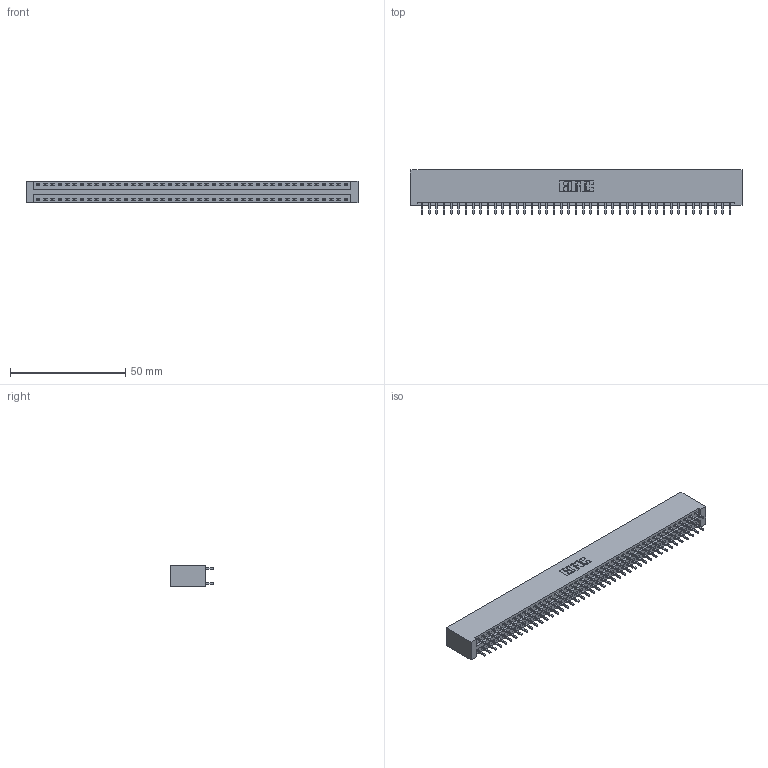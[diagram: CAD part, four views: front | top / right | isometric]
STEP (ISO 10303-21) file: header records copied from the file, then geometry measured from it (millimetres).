
FILE_DESCRIPTION (( 'STEP AP203' ), '1' );
FILE_NAME ('396-086-521-201.STEP', '2018-09-10T02:40:55', ( '' ), ( '' ), 'SwSTEP 2.0', 'SolidWorks 2016', '' );
FILE_SCHEMA (( 'CONFIG_CONTROL_DESIGN' ));
Length unit declared in the file: inch
Products named in the file (3): 346 Part_No Mounting Lugs; 345-292-001_345-293-121; 396-086-521-201
Assembly tree (87 placements, depth 2):
  396-086-521-201
    346 Part_No Mounting Lugs
    345-292-001_345-293-121  x86
Bounding box: 143.76 x 19.05 x 9.4 mm (x, y, z)
Volume: 14564.7 mm3; surface area: 19962.7 mm2
Topology: 87 solids, 87 shells, 4586 faces, 13635 edges, 8974 vertices
Faces by surface type: plane 3082, cylinder 1504
Entity records: 27669 total; most frequent: CARTESIAN_POINT 4556, ORIENTED_EDGE 4490, DIRECTION 4061, EDGE_CURVE 2245, VECTOR 1949, LINE 1949, VERTEX_POINT 1494, AXIS2_PLACEMENT_3D 1056
